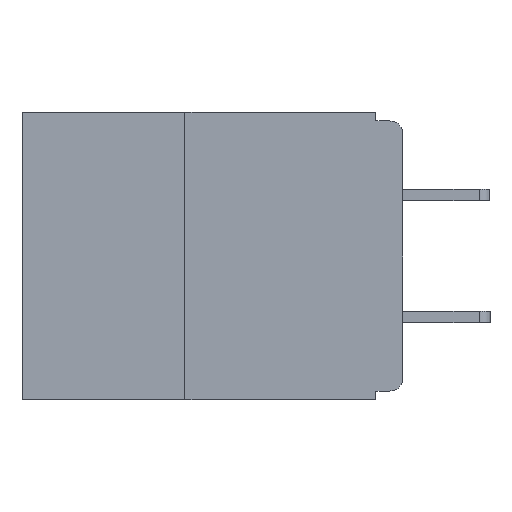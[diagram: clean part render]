
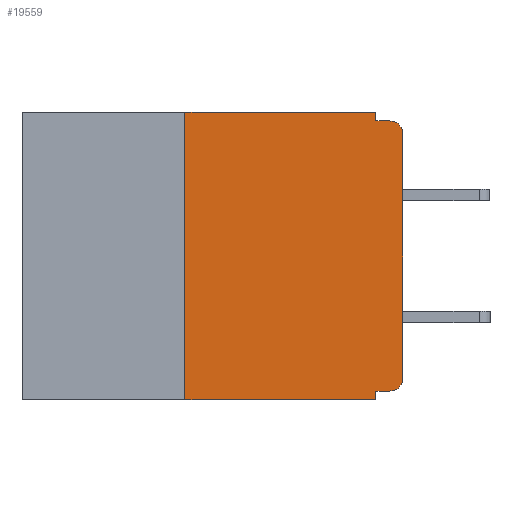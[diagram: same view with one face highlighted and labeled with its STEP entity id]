
A CAD part, left-side view. The second image highlights one B-rep face of the part: STEP entity #19559.
In plain terms, the highlighted planar face has unit normal (-1, 0, 0).
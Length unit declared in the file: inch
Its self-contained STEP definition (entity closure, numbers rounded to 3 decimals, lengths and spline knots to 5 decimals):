
#1043 = VERTEX_POINT ( 'NONE', #10011 ) ;
#1326 = CARTESIAN_POINT ( 'NONE',  ( 0., 0.437, 0. ) ) ;
#1569 = CARTESIAN_POINT ( 'NONE',  ( 0., 0.437, -0.33 ) ) ;
#1576 = EDGE_CURVE ( 'NONE', #1043, #20932, #16099, .T. ) ;
#1879 = LINE ( 'NONE', #5442, #16174 ) ;
#1904 = VERTEX_POINT ( 'NONE', #22691 ) ;
#2239 = AXIS2_PLACEMENT_3D ( 'NONE', #8988, #18201, #7162 ) ;
#2266 = VECTOR ( 'NONE', #16942, 39.37008 ) ;
#2409 = VECTOR ( 'NONE', #4353, 39.37008 ) ;
#2861 = LINE ( 'NONE', #17027, #2266 ) ;
#3116 = ORIENTED_EDGE ( 'NONE', *, *, #1576, .F. ) ;
#3992 = VERTEX_POINT ( 'NONE', #18904 ) ;
#4248 = ORIENTED_EDGE ( 'NONE', *, *, #5050, .F. ) ;
#4353 = DIRECTION ( 'NONE',  ( 0., 1., 0. ) ) ;
#5050 = EDGE_CURVE ( 'NONE', #19720, #15384, #2861, .T. ) ;
#5405 = ORIENTED_EDGE ( 'NONE', *, *, #18714, .T. ) ;
#5442 = CARTESIAN_POINT ( 'NONE',  ( 0., 0.25, -0.33 ) ) ;
#5597 = CARTESIAN_POINT ( 'NONE',  ( 0., 0., 0. ) ) ;
#5828 = CARTESIAN_POINT ( 'NONE',  ( 0., 0.015, -0.025 ) ) ;
#5911 = ORIENTED_EDGE ( 'NONE', *, *, #17546, .T. ) ;
#5925 = CARTESIAN_POINT ( 'NONE',  ( 0., 0.015, -0.305 ) ) ;
#5929 = ORIENTED_EDGE ( 'NONE', *, *, #10125, .F. ) ;
#6219 = CARTESIAN_POINT ( 'NONE',  ( 0., 0., -0.32 ) ) ;
#6267 = VECTOR ( 'NONE', #20512, 39.37008 ) ;
#6645 = VERTEX_POINT ( 'NONE', #12614 ) ;
#7162 = DIRECTION ( 'NONE',  ( 0., 0., -1. ) ) ;
#7294 = CIRCLE ( 'NONE', #18291, 0.015 ) ;
#7380 = EDGE_CURVE ( 'NONE', #15384, #3992, #17621, .T. ) ;
#7473 = ORIENTED_EDGE ( 'NONE', *, *, #7380, .F. ) ;
#7677 = DIRECTION ( 'NONE',  ( 0., 0., 1. ) ) ;
#7724 = DIRECTION ( 'NONE',  ( 0., 0., -1. ) ) ;
#7816 = DIRECTION ( 'NONE',  ( 0., 0., -1. ) ) ;
#8053 = CARTESIAN_POINT ( 'NONE',  ( 0., 0.25, 0. ) ) ;
#8313 = ORIENTED_EDGE ( 'NONE', *, *, #18204, .T. ) ;
#8663 = VERTEX_POINT ( 'NONE', #23111 ) ;
#8988 = CARTESIAN_POINT ( 'NONE',  ( 0., 0.437, 0. ) ) ;
#9006 = EDGE_CURVE ( 'NONE', #8663, #1904, #12228, .T. ) ;
#10011 = CARTESIAN_POINT ( 'NONE',  ( 0., 0.031, -0.32 ) ) ;
#10125 = EDGE_CURVE ( 'NONE', #6645, #12757, #1879, .T. ) ;
#10556 = ORIENTED_EDGE ( 'NONE', *, *, #9006, .T. ) ;
#10965 = EDGE_CURVE ( 'NONE', #8663, #1043, #17299, .T. ) ;
#11332 = VECTOR ( 'NONE', #18179, 39.37008 ) ;
#12158 = VECTOR ( 'NONE', #23176, 39.37008 ) ;
#12228 = CIRCLE ( 'NONE', #21451, 0.015 ) ;
#12614 = CARTESIAN_POINT ( 'NONE',  ( 0., 0.25, -0.33 ) ) ;
#12757 = VERTEX_POINT ( 'NONE', #8053 ) ;
#13288 = ORIENTED_EDGE ( 'NONE', *, *, #21901, .F. ) ;
#15369 = CARTESIAN_POINT ( 'NONE',  ( 0., 0., -0.025 ) ) ;
#15384 = VERTEX_POINT ( 'NONE', #20108 ) ;
#15678 = VECTOR ( 'NONE', #7677, 39.37008 ) ;
#16099 = LINE ( 'NONE', #22350, #6267 ) ;
#16174 = VECTOR ( 'NONE', #20252, 39.37008 ) ;
#16274 = PLANE ( 'NONE',  #2239 ) ;
#16809 = LINE ( 'NONE', #1326, #11332 ) ;
#16942 = DIRECTION ( 'NONE',  ( 0., 0., -1. ) ) ;
#17027 = CARTESIAN_POINT ( 'NONE',  ( 0., 0.031, 0. ) ) ;
#17299 = LINE ( 'NONE', #6219, #2409 ) ;
#17546 = EDGE_CURVE ( 'NONE', #1904, #19853, #20560, .T. ) ;
#17621 = LINE ( 'NONE', #23482, #12158 ) ;
#18151 = FACE_OUTER_BOUND ( 'NONE', #18357, .T. ) ;
#18179 = DIRECTION ( 'NONE',  ( 0., -1., 0. ) ) ;
#18201 = DIRECTION ( 'NONE',  ( 1., 0., 0. ) ) ;
#18204 = EDGE_CURVE ( 'NONE', #19853, #3992, #7294, .T. ) ;
#18291 = AXIS2_PLACEMENT_3D ( 'NONE', #5828, #18759, #7724 ) ;
#18333 = DIRECTION ( 'NONE',  ( 0., -1., 0. ) ) ;
#18357 = EDGE_LOOP ( 'NONE', ( #5911, #8313, #7473, #4248, #13288, #5929, #5405, #3116, #23128, #10556 ) ) ;
#18504 = VECTOR ( 'NONE', #18333, 39.37008 ) ;
#18714 = EDGE_CURVE ( 'NONE', #6645, #20932, #23196, .T. ) ;
#18759 = DIRECTION ( 'NONE',  ( -1., 0., 0. ) ) ;
#18850 = DIRECTION ( 'NONE',  ( -1., 0., 0. ) ) ;
#18904 = CARTESIAN_POINT ( 'NONE',  ( 0., 0.015, -0.01 ) ) ;
#19559 = ADVANCED_FACE ( 'NONE', ( #18151 ), #16274, .F. ) ;
#19720 = VERTEX_POINT ( 'NONE', #23822 ) ;
#19853 = VERTEX_POINT ( 'NONE', #15369 ) ;
#20108 = CARTESIAN_POINT ( 'NONE',  ( 0., 0.031, -0.01 ) ) ;
#20252 = DIRECTION ( 'NONE',  ( 0., 0., 1. ) ) ;
#20512 = DIRECTION ( 'NONE',  ( 0., 0., -1. ) ) ;
#20539 = CARTESIAN_POINT ( 'NONE',  ( 0., 0.031, -0.33 ) ) ;
#20560 = LINE ( 'NONE', #5597, #15678 ) ;
#20932 = VERTEX_POINT ( 'NONE', #20539 ) ;
#21451 = AXIS2_PLACEMENT_3D ( 'NONE', #5925, #18850, #7816 ) ;
#21901 = EDGE_CURVE ( 'NONE', #12757, #19720, #16809, .T. ) ;
#22350 = CARTESIAN_POINT ( 'NONE',  ( 0., 0.031, -0.33 ) ) ;
#22691 = CARTESIAN_POINT ( 'NONE',  ( 0., 0., -0.305 ) ) ;
#23111 = CARTESIAN_POINT ( 'NONE',  ( 0., 0.015, -0.32 ) ) ;
#23128 = ORIENTED_EDGE ( 'NONE', *, *, #10965, .F. ) ;
#23176 = DIRECTION ( 'NONE',  ( 0., -1., 0. ) ) ;
#23196 = LINE ( 'NONE', #1569, #18504 ) ;
#23482 = CARTESIAN_POINT ( 'NONE',  ( 0., 0., -0.01 ) ) ;
#23822 = CARTESIAN_POINT ( 'NONE',  ( 0., 0.031, 0. ) ) ;
